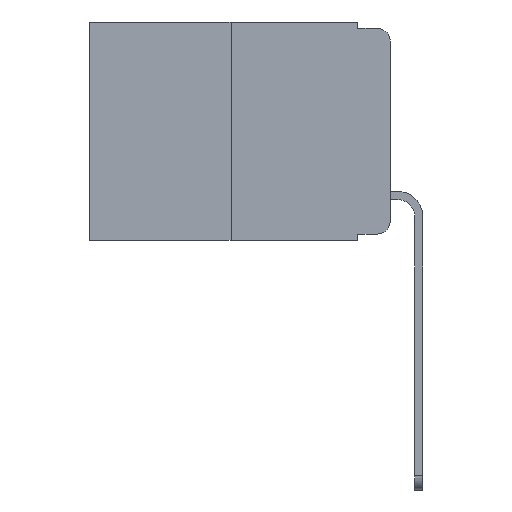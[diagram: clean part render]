
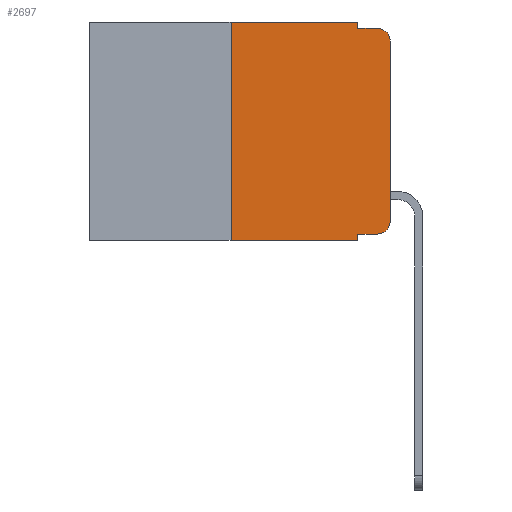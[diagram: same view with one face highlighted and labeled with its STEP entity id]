
A CAD part, left-side view. The second image highlights one B-rep face of the part: STEP entity #2697.
In plain terms, the highlighted planar face has unit normal (-1, 0, 0).
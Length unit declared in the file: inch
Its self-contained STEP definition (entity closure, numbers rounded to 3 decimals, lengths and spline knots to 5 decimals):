
#211 = CARTESIAN_POINT ( 'NONE',  ( 0., 0.02, -0.313 ) ) ;
#230 = CARTESIAN_POINT ( 'NONE',  ( 0., 0.051, -0.333 ) ) ;
#348 = EDGE_CURVE ( 'NONE', #8874, #6907, #8268, .T. ) ;
#1184 = DIRECTION ( 'NONE',  ( 0., 0., -1. ) ) ;
#1484 = CARTESIAN_POINT ( 'NONE',  ( 0., 0.051, -0.01 ) ) ;
#1537 = VERTEX_POINT ( 'NONE', #2210 ) ;
#1810 = VERTEX_POINT ( 'NONE', #4539 ) ;
#2143 = PLANE ( 'NONE',  #9148 ) ;
#2210 = CARTESIAN_POINT ( 'NONE',  ( 0., 0.051, -0.01 ) ) ;
#2592 = DIRECTION ( 'NONE',  ( 0., -1., 0. ) ) ;
#2697 = ADVANCED_FACE ( 'NONE', ( #4348 ), #2143, .F. ) ;
#2739 = CARTESIAN_POINT ( 'NONE',  ( 0., 0.051, 0. ) ) ;
#2890 = CARTESIAN_POINT ( 'NONE',  ( 0., 0.473, -0.343 ) ) ;
#2963 = VECTOR ( 'NONE', #12700, 39.37008 ) ;
#3399 = LINE ( 'NONE', #5508, #8325 ) ;
#3422 = EDGE_CURVE ( 'NONE', #7105, #8761, #9101, .T. ) ;
#3605 = VECTOR ( 'NONE', #2592, 39.37008 ) ;
#3621 = VERTEX_POINT ( 'NONE', #10375 ) ;
#3659 = EDGE_CURVE ( 'NONE', #1810, #12711, #6320, .T. ) ;
#3777 = CARTESIAN_POINT ( 'NONE',  ( 0., 0.051, -0.343 ) ) ;
#4348 = FACE_OUTER_BOUND ( 'NONE', #7521, .T. ) ;
#4539 = CARTESIAN_POINT ( 'NONE',  ( 0., 0., -0.03 ) ) ;
#4561 = CARTESIAN_POINT ( 'NONE',  ( 0., 0.02, -0.03 ) ) ;
#4731 = CARTESIAN_POINT ( 'NONE',  ( 0., 0., 0. ) ) ;
#4837 = ORIENTED_EDGE ( 'NONE', *, *, #7694, .F. ) ;
#4940 = ORIENTED_EDGE ( 'NONE', *, *, #10200, .T. ) ;
#5043 = ORIENTED_EDGE ( 'NONE', *, *, #12596, .T. ) ;
#5053 = EDGE_CURVE ( 'NONE', #3621, #7398, #3399, .T. ) ;
#5129 = DIRECTION ( 'NONE',  ( 1., 0., 0. ) ) ;
#5189 = CARTESIAN_POINT ( 'NONE',  ( 0., 0.25, 0. ) ) ;
#5275 = LINE ( 'NONE', #2890, #2963 ) ;
#5508 = CARTESIAN_POINT ( 'NONE',  ( 0., 0.051, 0. ) ) ;
#5542 = DIRECTION ( 'NONE',  ( 0., 0., -1. ) ) ;
#5649 = VECTOR ( 'NONE', #8145, 39.37008 ) ;
#5938 = CARTESIAN_POINT ( 'NONE',  ( 0., 0.25, 0. ) ) ;
#6233 = CARTESIAN_POINT ( 'NONE',  ( 0., 0.02, -0.333 ) ) ;
#6320 = CIRCLE ( 'NONE', #10408, 0.02 ) ;
#6402 = DIRECTION ( 'NONE',  ( 0., -1., 0. ) ) ;
#6506 = DIRECTION ( 'NONE',  ( 0., 0., -1. ) ) ;
#6626 = VERTEX_POINT ( 'NONE', #7490 ) ;
#6907 = VERTEX_POINT ( 'NONE', #5938 ) ;
#7103 = DIRECTION ( 'NONE',  ( -1., 0., 0. ) ) ;
#7105 = VERTEX_POINT ( 'NONE', #6233 ) ;
#7126 = DIRECTION ( 'NONE',  ( 0., -1., 0. ) ) ;
#7398 = VERTEX_POINT ( 'NONE', #3777 ) ;
#7428 = LINE ( 'NONE', #2739, #7730 ) ;
#7490 = CARTESIAN_POINT ( 'NONE',  ( 0., 0.051, 0. ) ) ;
#7521 = EDGE_LOOP ( 'NONE', ( #9559, #11216, #4837, #8730, #10769, #9177, #5043, #10625, #4940, #9876 ) ) ;
#7694 = EDGE_CURVE ( 'NONE', #1537, #12711, #8923, .T. ) ;
#7730 = VECTOR ( 'NONE', #12581, 39.37008 ) ;
#8145 = DIRECTION ( 'NONE',  ( 0., 0., 1. ) ) ;
#8268 = LINE ( 'NONE', #5189, #5649 ) ;
#8325 = VECTOR ( 'NONE', #6506, 39.37008 ) ;
#8730 = ORIENTED_EDGE ( 'NONE', *, *, #11720, .F. ) ;
#8761 = VERTEX_POINT ( 'NONE', #8960 ) ;
#8874 = VERTEX_POINT ( 'NONE', #9078 ) ;
#8923 = LINE ( 'NONE', #1484, #10623 ) ;
#8960 = CARTESIAN_POINT ( 'NONE',  ( 0., 0., -0.313 ) ) ;
#9032 = CARTESIAN_POINT ( 'NONE',  ( 0., 0.473, 0. ) ) ;
#9078 = CARTESIAN_POINT ( 'NONE',  ( 0., 0.25, -0.343 ) ) ;
#9101 = CIRCLE ( 'NONE', #11953, 0.02 ) ;
#9148 = AXIS2_PLACEMENT_3D ( 'NONE', #9032, #5129, #11999 ) ;
#9177 = ORIENTED_EDGE ( 'NONE', *, *, #348, .F. ) ;
#9559 = ORIENTED_EDGE ( 'NONE', *, *, #11705, .T. ) ;
#9635 = VECTOR ( 'NONE', #7126, 39.37008 ) ;
#9738 = VECTOR ( 'NONE', #10617, 39.37008 ) ;
#9876 = ORIENTED_EDGE ( 'NONE', *, *, #3422, .T. ) ;
#10200 = EDGE_CURVE ( 'NONE', #3621, #7105, #11613, .T. ) ;
#10375 = CARTESIAN_POINT ( 'NONE',  ( 0., 0.051, -0.333 ) ) ;
#10408 = AXIS2_PLACEMENT_3D ( 'NONE', #4561, #11421, #5542 ) ;
#10428 = EDGE_CURVE ( 'NONE', #6907, #6626, #11448, .T. ) ;
#10477 = CARTESIAN_POINT ( 'NONE',  ( 0., 0.473, 0. ) ) ;
#10617 = DIRECTION ( 'NONE',  ( 0., 0., 1. ) ) ;
#10623 = VECTOR ( 'NONE', #6402, 39.37008 ) ;
#10625 = ORIENTED_EDGE ( 'NONE', *, *, #5053, .F. ) ;
#10769 = ORIENTED_EDGE ( 'NONE', *, *, #10428, .F. ) ;
#11216 = ORIENTED_EDGE ( 'NONE', *, *, #3659, .T. ) ;
#11421 = DIRECTION ( 'NONE',  ( -1., 0., 0. ) ) ;
#11448 = LINE ( 'NONE', #10477, #3605 ) ;
#11613 = LINE ( 'NONE', #230, #9635 ) ;
#11705 = EDGE_CURVE ( 'NONE', #8761, #1810, #12341, .T. ) ;
#11720 = EDGE_CURVE ( 'NONE', #6626, #1537, #7428, .T. ) ;
#11879 = CARTESIAN_POINT ( 'NONE',  ( 0., 0.02, -0.01 ) ) ;
#11953 = AXIS2_PLACEMENT_3D ( 'NONE', #211, #7103, #1184 ) ;
#11999 = DIRECTION ( 'NONE',  ( 0., 0., -1. ) ) ;
#12341 = LINE ( 'NONE', #4731, #9738 ) ;
#12581 = DIRECTION ( 'NONE',  ( 0., 0., -1. ) ) ;
#12596 = EDGE_CURVE ( 'NONE', #8874, #7398, #5275, .T. ) ;
#12700 = DIRECTION ( 'NONE',  ( 0., -1., 0. ) ) ;
#12711 = VERTEX_POINT ( 'NONE', #11879 ) ;
